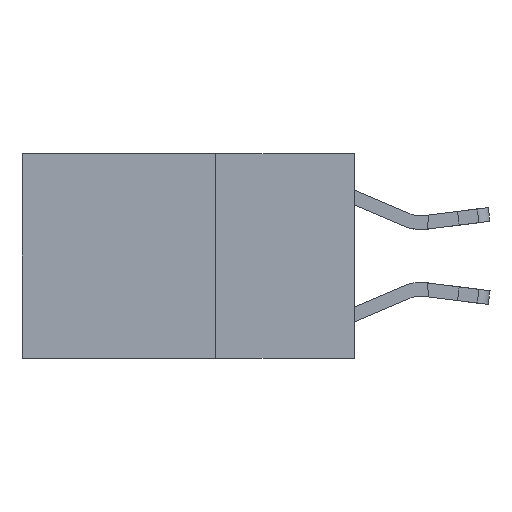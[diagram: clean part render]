
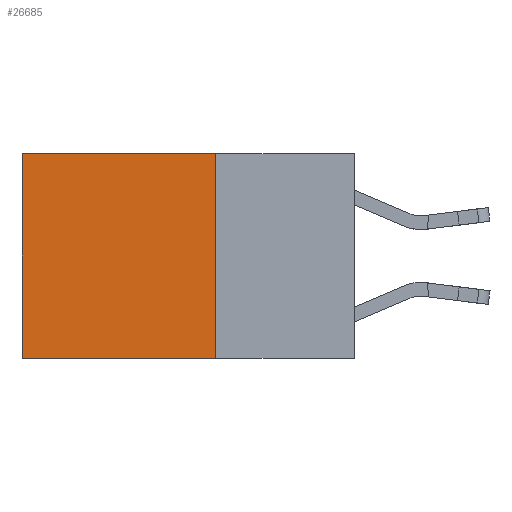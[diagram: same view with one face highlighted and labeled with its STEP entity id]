
A CAD part, left-side view. The second image highlights one B-rep face of the part: STEP entity #26685.
In plain terms, the highlighted planar face has unit normal (-1, 0, 0).
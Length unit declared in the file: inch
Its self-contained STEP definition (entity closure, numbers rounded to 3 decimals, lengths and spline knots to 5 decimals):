
#288 = ORIENTED_EDGE ( 'NONE', *, *, #2001, .F. ) ;
#1145 = VECTOR ( 'NONE', #4565, 39.37008 ) ;
#1691 = VERTEX_POINT ( 'NONE', #13279 ) ;
#1780 = LINE ( 'NONE', #14327, #13416 ) ;
#2001 = EDGE_CURVE ( 'NONE', #1691, #11229, #7286, .T. ) ;
#3149 = DIRECTION ( 'NONE',  ( 0., 1., 0. ) ) ;
#4565 = DIRECTION ( 'NONE',  ( 0., 0., -1. ) ) ;
#6888 = EDGE_LOOP ( 'NONE', ( #21196, #288, #24818, #17908 ) ) ;
#7286 = LINE ( 'NONE', #13175, #22167 ) ;
#9109 = DIRECTION ( 'NONE',  ( 1., 0., 0. ) ) ;
#9140 = AXIS2_PLACEMENT_3D ( 'NONE', #21749, #9109, #11530 ) ;
#9745 = VERTEX_POINT ( 'NONE', #23336 ) ;
#10438 = DIRECTION ( 'NONE',  ( 0., 0., -1. ) ) ;
#10504 = VERTEX_POINT ( 'NONE', #11001 ) ;
#10961 = EDGE_CURVE ( 'NONE', #9745, #1691, #1780, .T. ) ;
#11001 = CARTESIAN_POINT ( 'NONE',  ( 0.2625, 0.6, 0. ) ) ;
#11055 = LINE ( 'NONE', #21003, #12019 ) ;
#11169 = EDGE_CURVE ( 'NONE', #10504, #11229, #16296, .T. ) ;
#11229 = VERTEX_POINT ( 'NONE', #23615 ) ;
#11530 = DIRECTION ( 'NONE',  ( 0., 0., -1. ) ) ;
#12019 = VECTOR ( 'NONE', #21174, 39.37008 ) ;
#12798 = CARTESIAN_POINT ( 'NONE',  ( 0.2625, 0.6, 0. ) ) ;
#13175 = CARTESIAN_POINT ( 'NONE',  ( 0.2625, 0.25, -0.37 ) ) ;
#13279 = CARTESIAN_POINT ( 'NONE',  ( 0.2625, 0.25, -0.37 ) ) ;
#13416 = VECTOR ( 'NONE', #10438, 39.37008 ) ;
#14327 = CARTESIAN_POINT ( 'NONE',  ( 0.2625, 0.25, 0. ) ) ;
#15695 = PLANE ( 'NONE',  #9140 ) ;
#16296 = LINE ( 'NONE', #12798, #1145 ) ;
#17908 = ORIENTED_EDGE ( 'NONE', *, *, #25843, .T. ) ;
#21003 = CARTESIAN_POINT ( 'NONE',  ( 0.2625, 0.25, 0. ) ) ;
#21174 = DIRECTION ( 'NONE',  ( 0., 1., 0. ) ) ;
#21196 = ORIENTED_EDGE ( 'NONE', *, *, #11169, .T. ) ;
#21749 = CARTESIAN_POINT ( 'NONE',  ( 0.2625, 0.25, 0. ) ) ;
#22167 = VECTOR ( 'NONE', #3149, 39.37008 ) ;
#23336 = CARTESIAN_POINT ( 'NONE',  ( 0.2625, 0.25, 0. ) ) ;
#23615 = CARTESIAN_POINT ( 'NONE',  ( 0.2625, 0.6, -0.37 ) ) ;
#23630 = FACE_OUTER_BOUND ( 'NONE', #6888, .T. ) ;
#24818 = ORIENTED_EDGE ( 'NONE', *, *, #10961, .F. ) ;
#25843 = EDGE_CURVE ( 'NONE', #9745, #10504, #11055, .T. ) ;
#26685 = ADVANCED_FACE ( 'NONE', ( #23630 ), #15695, .F. ) ;
